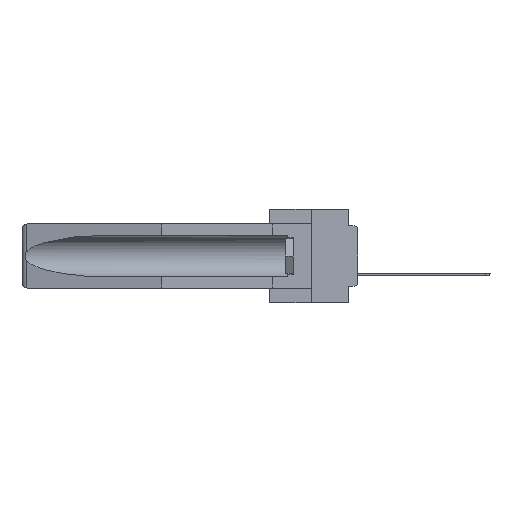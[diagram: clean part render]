
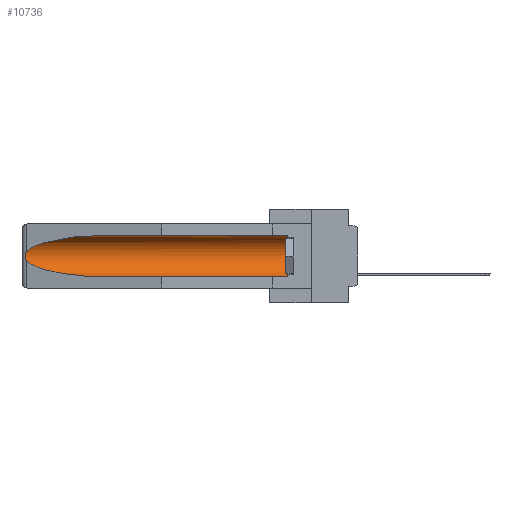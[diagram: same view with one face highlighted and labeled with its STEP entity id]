
A CAD part, left-side view. The second image highlights one B-rep face of the part: STEP entity #10736.
In plain terms, the highlighted cylindrical face has radius 2.857 mm (diameter 5.715 mm), a partial arc.
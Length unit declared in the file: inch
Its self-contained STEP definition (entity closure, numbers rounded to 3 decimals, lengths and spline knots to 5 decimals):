
#106 = CARTESIAN_POINT ( 'NONE',  ( 0.26654, 1.53092, -0.15636 ) ) ;
#1227 = CIRCLE ( 'NONE', #13666, 0.1125 ) ;
#1271 = CARTESIAN_POINT ( 'NONE',  ( 0.25451, 1.48313, -0.24835 ) ) ;
#1411 = CARTESIAN_POINT ( 'NONE',  ( 0.155, 1.07973, -0.059 ) ) ;
#3069 = CARTESIAN_POINT ( 'NONE',  ( 0.155, -0.30754, -0.059 ) ) ;
#3126 =( BOUNDED_CURVE ( )  B_SPLINE_CURVE ( 3, ( #1411, #15348, #3658, #14896 ),
 .UNSPECIFIED., .F., .F. ) 
 B_SPLINE_CURVE_WITH_KNOTS ( ( 4, 4 ),
 ( 4.71239, 6.08839 ),
 .UNSPECIFIED. ) 
 CURVE ( )  GEOMETRIC_REPRESENTATION_ITEM ( )  RATIONAL_B_SPLINE_CURVE ( ( 1., 0.848, 0.848, 1. ) ) 
 REPRESENTATION_ITEM ( '' )  );
#3223 = EDGE_CURVE ( 'NONE', #27518, #21713, #25574, .T. ) ;
#3658 = CARTESIAN_POINT ( 'NONE',  ( 0.25451, 1.48313, -0.09465 ) ) ;
#3928 =( BOUNDED_CURVE ( )  B_SPLINE_CURVE ( 3, ( #6211, #1271, #15211, #19843 ),
 .UNSPECIFIED., .F., .F. ) 
 B_SPLINE_CURVE_WITH_KNOTS ( ( 4, 4 ),
 ( 0.1948, 1.5708 ),
 .UNSPECIFIED. ) 
 CURVE ( )  GEOMETRIC_REPRESENTATION_ITEM ( )  RATIONAL_B_SPLINE_CURVE ( ( 1., 0.848, 0.848, 1. ) ) 
 REPRESENTATION_ITEM ( '' )  );
#4399 = EDGE_CURVE ( 'NONE', #13495, #28038, #27248, .T. ) ;
#5026 = DIRECTION ( 'NONE',  ( 0., 1., 0. ) ) ;
#5142 = EDGE_CURVE ( 'NONE', #22466, #13495, #3126, .T. ) ;
#5162 = DIRECTION ( 'NONE',  ( 0., 1., 0. ) ) ;
#5220 = ORIENTED_EDGE ( 'NONE', *, *, #14901, .T. ) ;
#5378 = DIRECTION ( 'NONE',  ( 0., -1., 0. ) ) ;
#6211 = CARTESIAN_POINT ( 'NONE',  ( 0.26537, 1.52718, -0.19328 ) ) ;
#6465 = CYLINDRICAL_SURFACE ( 'NONE', #17306, 0.1125 ) ;
#6858 = ORIENTED_EDGE ( 'NONE', *, *, #5142, .T. ) ;
#7727 = ORIENTED_EDGE ( 'NONE', *, *, #4399, .T. ) ;
#7845 = LINE ( 'NONE', #3069, #12476 ) ;
#8270 = CARTESIAN_POINT ( 'NONE',  ( 0.155, 0.126, -0.284 ) ) ;
#8904 = VERTEX_POINT ( 'NONE', #21932 ) ;
#8953 = CARTESIAN_POINT ( 'NONE',  ( 0.2675, 1.53308, -0.17534 ) ) ;
#9575 = CARTESIAN_POINT ( 'NONE',  ( 0.155, 0.126, -0.1715 ) ) ;
#9979 = EDGE_LOOP ( 'NONE', ( #6858, #7727, #20997, #12596, #5220, #13322 ) ) ;
#10079 = EDGE_CURVE ( 'NONE', #8904, #22466, #7845, .T. ) ;
#10736 = ADVANCED_FACE ( 'NONE', ( #22351 ), #6465, .F. ) ;
#11812 = CARTESIAN_POINT ( 'NONE',  ( 0.155, 1.07973, -0.284 ) ) ;
#11924 = CARTESIAN_POINT ( 'NONE',  ( 0.155, -0.30754, -0.284 ) ) ;
#12476 = VECTOR ( 'NONE', #5162, 39.37008 ) ;
#12596 = ORIENTED_EDGE ( 'NONE', *, *, #3223, .F. ) ;
#13322 = ORIENTED_EDGE ( 'NONE', *, *, #10079, .T. ) ;
#13495 = VERTEX_POINT ( 'NONE', #25030 ) ;
#13666 = AXIS2_PLACEMENT_3D ( 'NONE', #9575, #5378, #28324 ) ;
#13744 = CARTESIAN_POINT ( 'NONE',  ( 0.26597, 1.52961, -0.15275 ) ) ;
#14190 = CARTESIAN_POINT ( 'NONE',  ( 0.26537, 1.52718, -0.19328 ) ) ;
#14215 = VECTOR ( 'NONE', #5026, 39.37008 ) ;
#14896 = CARTESIAN_POINT ( 'NONE',  ( 0.26537, 1.52718, -0.14972 ) ) ;
#14901 = EDGE_CURVE ( 'NONE', #27518, #8904, #1227, .T. ) ;
#15211 = CARTESIAN_POINT ( 'NONE',  ( 0.21114, 1.30732, -0.284 ) ) ;
#15348 = CARTESIAN_POINT ( 'NONE',  ( 0.21114, 1.30732, -0.059 ) ) ;
#16298 = CARTESIAN_POINT ( 'NONE',  ( 0.2673, 1.5327, -0.16383 ) ) ;
#17306 = AXIS2_PLACEMENT_3D ( 'NONE', #22798, #20255, #18152 ) ;
#18152 = DIRECTION ( 'NONE',  ( 0., 0., 1. ) ) ;
#19843 = CARTESIAN_POINT ( 'NONE',  ( 0.155, 1.07973, -0.284 ) ) ;
#20255 = DIRECTION ( 'NONE',  ( 0., 1., 0. ) ) ;
#20486 = CARTESIAN_POINT ( 'NONE',  ( 0.26655, 1.53094, -0.18657 ) ) ;
#20634 = CARTESIAN_POINT ( 'NONE',  ( 0.26537, 1.52718, -0.14972 ) ) ;
#20664 = CARTESIAN_POINT ( 'NONE',  ( 0.26597, 1.5296, -0.19026 ) ) ;
#20772 = CARTESIAN_POINT ( 'NONE',  ( 0.2673, 1.53269, -0.17917 ) ) ;
#20923 = CARTESIAN_POINT ( 'NONE',  ( 0.2675, 1.53308, -0.16763 ) ) ;
#20997 = ORIENTED_EDGE ( 'NONE', *, *, #27070, .T. ) ;
#21713 = VERTEX_POINT ( 'NONE', #11812 ) ;
#21932 = CARTESIAN_POINT ( 'NONE',  ( 0.155, 0.126, -0.059 ) ) ;
#22351 = FACE_OUTER_BOUND ( 'NONE', #9979, .T. ) ;
#22466 = VERTEX_POINT ( 'NONE', #29600 ) ;
#22798 = CARTESIAN_POINT ( 'NONE',  ( 0.155, -0.30754, -0.1715 ) ) ;
#22890 = CARTESIAN_POINT ( 'NONE',  ( 0.26537, 1.52718, -0.19328 ) ) ;
#25030 = CARTESIAN_POINT ( 'NONE',  ( 0.26537, 1.52718, -0.14972 ) ) ;
#25574 = LINE ( 'NONE', #11924, #14215 ) ;
#27070 = EDGE_CURVE ( 'NONE', #28038, #21713, #3928, .T. ) ;
#27248 = B_SPLINE_CURVE_WITH_KNOTS ( 'NONE', 3,
 ( #20634, #13744, #106, #16298, #20923, #8953, #20772, #20486, #20664, #22890 ),
 .UNSPECIFIED., .F., .F.,
 ( 4, 2, 2, 2, 4 ),
 ( 0., 0.00029, 0.00058, 0.00087, 0.00117 ),
 .UNSPECIFIED. ) ;
#27518 = VERTEX_POINT ( 'NONE', #8270 ) ;
#28038 = VERTEX_POINT ( 'NONE', #14190 ) ;
#28324 = DIRECTION ( 'NONE',  ( 0., 0., 1. ) ) ;
#29600 = CARTESIAN_POINT ( 'NONE',  ( 0.155, 1.07973, -0.059 ) ) ;
